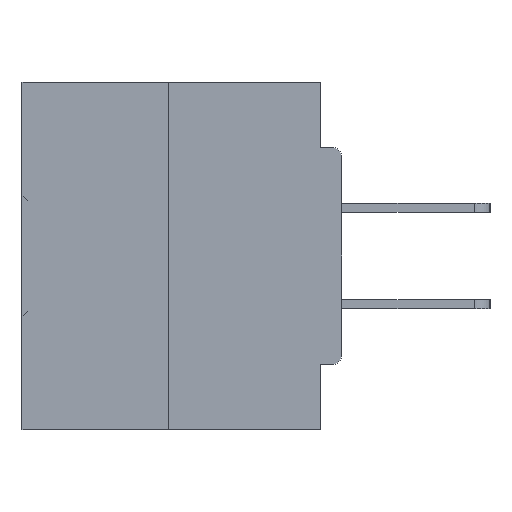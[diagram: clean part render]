
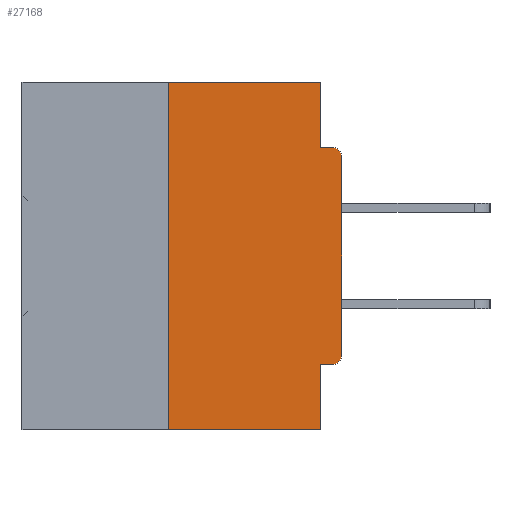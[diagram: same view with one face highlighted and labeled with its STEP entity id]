
A CAD part, left-side view. The second image highlights one B-rep face of the part: STEP entity #27168.
In plain terms, the highlighted planar face has unit normal (-1, 0, 0).
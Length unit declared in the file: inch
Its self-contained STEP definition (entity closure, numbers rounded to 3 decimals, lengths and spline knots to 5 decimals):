
#590 = DIRECTION ( 'NONE',  ( 0., 0., -1. ) ) ;
#991 = EDGE_CURVE ( 'NONE', #33068, #38646, #23242, .T. ) ;
#2225 = AXIS2_PLACEMENT_3D ( 'NONE', #25896, #22343, #590 ) ;
#2319 = LINE ( 'NONE', #44255, #42395 ) ;
#2753 = CARTESIAN_POINT ( 'NONE',  ( 0., 0., -0.0935 ) ) ;
#2835 = DIRECTION ( 'NONE',  ( 0., -1., 0. ) ) ;
#3033 = LINE ( 'NONE', #13987, #23007 ) ;
#5281 = CARTESIAN_POINT ( 'NONE',  ( 0., 0.015, -0.0935 ) ) ;
#6185 = CARTESIAN_POINT ( 'NONE',  ( 0., 0.031, 0. ) ) ;
#6584 = FACE_OUTER_BOUND ( 'NONE', #22785, .T. ) ;
#7542 = ORIENTED_EDGE ( 'NONE', *, *, #21086, .F. ) ;
#7741 = DIRECTION ( 'NONE',  ( 0., -1., 0. ) ) ;
#8063 = DIRECTION ( 'NONE',  ( -1., 0., 0. ) ) ;
#9349 = AXIS2_PLACEMENT_3D ( 'NONE', #17179, #24069, #35195 ) ;
#9469 = EDGE_CURVE ( 'NONE', #32305, #30059, #22203, .T. ) ;
#10555 = VECTOR ( 'NONE', #34312, 39.37008 ) ;
#10692 = CARTESIAN_POINT ( 'NONE',  ( 0., 0., -0.1085 ) ) ;
#11092 = CARTESIAN_POINT ( 'NONE',  ( 0., 0.25, -0.5 ) ) ;
#12335 = ORIENTED_EDGE ( 'NONE', *, *, #14193, .F. ) ;
#12492 = CARTESIAN_POINT ( 'NONE',  ( 0., 0.015, -0.4065 ) ) ;
#13543 = VERTEX_POINT ( 'NONE', #6185 ) ;
#13580 = DIRECTION ( 'NONE',  ( 0., 0., -1. ) ) ;
#13987 = CARTESIAN_POINT ( 'NONE',  ( 0., 0.46, 0. ) ) ;
#14193 = EDGE_CURVE ( 'NONE', #19363, #18585, #30851, .T. ) ;
#15194 = ORIENTED_EDGE ( 'NONE', *, *, #19449, .F. ) ;
#15235 = CARTESIAN_POINT ( 'NONE',  ( 0., 0.015, -0.3915 ) ) ;
#15420 = CARTESIAN_POINT ( 'NONE',  ( 0., 0., -0.3915 ) ) ;
#15720 = CIRCLE ( 'NONE', #2225, 0.015 ) ;
#17179 = CARTESIAN_POINT ( 'NONE',  ( 0., 0.46, 0. ) ) ;
#17252 = ORIENTED_EDGE ( 'NONE', *, *, #24134, .T. ) ;
#17821 = VECTOR ( 'NONE', #46276, 39.37008 ) ;
#18585 = VERTEX_POINT ( 'NONE', #32900 ) ;
#19363 = VERTEX_POINT ( 'NONE', #24427 ) ;
#19449 = EDGE_CURVE ( 'NONE', #38646, #13543, #3033, .T. ) ;
#21086 = EDGE_CURVE ( 'NONE', #32305, #19363, #37363, .T. ) ;
#21374 = ORIENTED_EDGE ( 'NONE', *, *, #33308, .F. ) ;
#21794 = VECTOR ( 'NONE', #38179, 39.37008 ) ;
#22203 = CIRCLE ( 'NONE', #27028, 0.015 ) ;
#22343 = DIRECTION ( 'NONE',  ( -1., 0., 0. ) ) ;
#22785 = EDGE_LOOP ( 'NONE', ( #15194, #31453, #30302, #12335, #7542, #45984, #42261, #17252, #21374, #43348 ) ) ;
#23007 = VECTOR ( 'NONE', #2835, 39.37008 ) ;
#23242 = LINE ( 'NONE', #34199, #30713 ) ;
#24069 = DIRECTION ( 'NONE',  ( 1., 0., 0. ) ) ;
#24134 = EDGE_CURVE ( 'NONE', #46593, #34174, #15720, .T. ) ;
#24427 = CARTESIAN_POINT ( 'NONE',  ( 0., 0.031, -0.4065 ) ) ;
#25469 = LINE ( 'NONE', #2753, #35272 ) ;
#25896 = CARTESIAN_POINT ( 'NONE',  ( 0., 0.015, -0.1085 ) ) ;
#26816 = VECTOR ( 'NONE', #13580, 39.37008 ) ;
#27028 = AXIS2_PLACEMENT_3D ( 'NONE', #15235, #8063, #29969 ) ;
#27168 = ADVANCED_FACE ( 'NONE', ( #6584 ), #39179, .F. ) ;
#27472 = CARTESIAN_POINT ( 'NONE',  ( 0., 0.031, 0. ) ) ;
#27473 = EDGE_CURVE ( 'NONE', #30059, #46593, #43784, .T. ) ;
#29969 = DIRECTION ( 'NONE',  ( 0., 0., -1. ) ) ;
#30059 = VERTEX_POINT ( 'NONE', #15420 ) ;
#30302 = ORIENTED_EDGE ( 'NONE', *, *, #31258, .T. ) ;
#30713 = VECTOR ( 'NONE', #41553, 39.37008 ) ;
#30851 = LINE ( 'NONE', #46635, #26816 ) ;
#31258 = EDGE_CURVE ( 'NONE', #33068, #18585, #2319, .T. ) ;
#31453 = ORIENTED_EDGE ( 'NONE', *, *, #991, .F. ) ;
#31611 = LINE ( 'NONE', #27472, #17821 ) ;
#32305 = VERTEX_POINT ( 'NONE', #12492 ) ;
#32900 = CARTESIAN_POINT ( 'NONE',  ( 0., 0.031, -0.5 ) ) ;
#33068 = VERTEX_POINT ( 'NONE', #11092 ) ;
#33308 = EDGE_CURVE ( 'NONE', #36687, #34174, #25469, .T. ) ;
#33982 = CARTESIAN_POINT ( 'NONE',  ( 0., 0., 0. ) ) ;
#34174 = VERTEX_POINT ( 'NONE', #5281 ) ;
#34199 = CARTESIAN_POINT ( 'NONE',  ( 0., 0.25, 0. ) ) ;
#34312 = DIRECTION ( 'NONE',  ( 0., 0., 1. ) ) ;
#35195 = DIRECTION ( 'NONE',  ( 0., 0., -1. ) ) ;
#35272 = VECTOR ( 'NONE', #46495, 39.37008 ) ;
#35661 = CARTESIAN_POINT ( 'NONE',  ( 0., 0.031, -0.0935 ) ) ;
#36687 = VERTEX_POINT ( 'NONE', #35661 ) ;
#37363 = LINE ( 'NONE', #45829, #21794 ) ;
#38179 = DIRECTION ( 'NONE',  ( 0., 1., 0. ) ) ;
#38646 = VERTEX_POINT ( 'NONE', #46859 ) ;
#39179 = PLANE ( 'NONE',  #9349 ) ;
#39515 = EDGE_CURVE ( 'NONE', #13543, #36687, #31611, .T. ) ;
#41553 = DIRECTION ( 'NONE',  ( 0., 0., 1. ) ) ;
#42261 = ORIENTED_EDGE ( 'NONE', *, *, #27473, .T. ) ;
#42395 = VECTOR ( 'NONE', #7741, 39.37008 ) ;
#43348 = ORIENTED_EDGE ( 'NONE', *, *, #39515, .F. ) ;
#43784 = LINE ( 'NONE', #33982, #10555 ) ;
#44255 = CARTESIAN_POINT ( 'NONE',  ( 0., 0.46, -0.5 ) ) ;
#45829 = CARTESIAN_POINT ( 'NONE',  ( 0., 0., -0.4065 ) ) ;
#45984 = ORIENTED_EDGE ( 'NONE', *, *, #9469, .T. ) ;
#46276 = DIRECTION ( 'NONE',  ( 0., 0., -1. ) ) ;
#46495 = DIRECTION ( 'NONE',  ( 0., -1., 0. ) ) ;
#46593 = VERTEX_POINT ( 'NONE', #10692 ) ;
#46635 = CARTESIAN_POINT ( 'NONE',  ( 0., 0.031, -0.5 ) ) ;
#46859 = CARTESIAN_POINT ( 'NONE',  ( 0., 0.25, 0. ) ) ;
